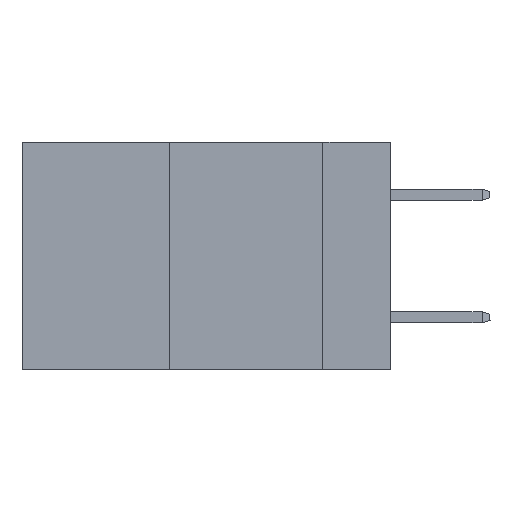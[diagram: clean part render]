
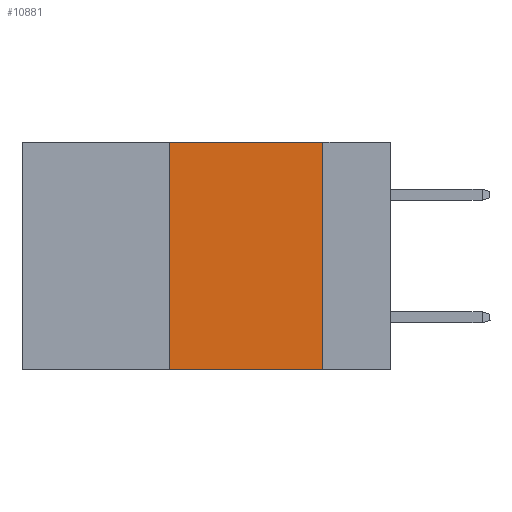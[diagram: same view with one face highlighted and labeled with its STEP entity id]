
A CAD part, left-side view. The second image highlights one B-rep face of the part: STEP entity #10881.
In plain terms, the highlighted planar face has unit normal (-1, 0, 0).
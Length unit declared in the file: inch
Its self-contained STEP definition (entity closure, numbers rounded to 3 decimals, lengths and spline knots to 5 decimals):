
#138 = DIRECTION ( 'NONE',  ( 0., -1., 0. ) ) ;
#1046 = DIRECTION ( 'NONE',  ( 0., -1., 0. ) ) ;
#1089 = VERTEX_POINT ( 'NONE', #20756 ) ;
#2280 = VERTEX_POINT ( 'NONE', #20161 ) ;
#2423 = EDGE_CURVE ( 'NONE', #1089, #2280, #5255, .T. ) ;
#2835 = PLANE ( 'NONE',  #19701 ) ;
#4960 = LINE ( 'NONE', #23471, #11288 ) ;
#5255 = LINE ( 'NONE', #24711, #20004 ) ;
#8834 = DIRECTION ( 'NONE',  ( 1., 0., 0. ) ) ;
#9177 = ORIENTED_EDGE ( 'NONE', *, *, #2423, .F. ) ;
#9410 = DIRECTION ( 'NONE',  ( 0., 0., 1. ) ) ;
#10291 = EDGE_CURVE ( 'NONE', #25453, #2280, #19579, .T. ) ;
#10881 = ADVANCED_FACE ( 'NONE', ( #21775 ), #2835, .F. ) ;
#11288 = VECTOR ( 'NONE', #9410, 39.37008 ) ;
#11901 = CARTESIAN_POINT ( 'NONE',  ( 0., 0.6, 0. ) ) ;
#12228 = ORIENTED_EDGE ( 'NONE', *, *, #10291, .T. ) ;
#12396 = LINE ( 'NONE', #11901, #24293 ) ;
#12636 = EDGE_LOOP ( 'NONE', ( #9177, #16327, #13466, #12228 ) ) ;
#13466 = ORIENTED_EDGE ( 'NONE', *, *, #22051, .F. ) ;
#16327 = ORIENTED_EDGE ( 'NONE', *, *, #21061, .F. ) ;
#16903 = CARTESIAN_POINT ( 'NONE',  ( 0., 0.6, 0. ) ) ;
#19579 = LINE ( 'NONE', #21078, #21771 ) ;
#19701 = AXIS2_PLACEMENT_3D ( 'NONE', #16903, #8834, #24838 ) ;
#20004 = VECTOR ( 'NONE', #24361, 39.37008 ) ;
#20161 = CARTESIAN_POINT ( 'NONE',  ( 0., 0.11, -0.37 ) ) ;
#20756 = CARTESIAN_POINT ( 'NONE',  ( 0., 0.11, 0. ) ) ;
#21061 = EDGE_CURVE ( 'NONE', #24851, #1089, #12396, .T. ) ;
#21078 = CARTESIAN_POINT ( 'NONE',  ( 0., 0.6, -0.37 ) ) ;
#21771 = VECTOR ( 'NONE', #1046, 39.37008 ) ;
#21775 = FACE_OUTER_BOUND ( 'NONE', #12636, .T. ) ;
#21942 = CARTESIAN_POINT ( 'NONE',  ( 0., 0.36, -0.37 ) ) ;
#22051 = EDGE_CURVE ( 'NONE', #25453, #24851, #4960, .T. ) ;
#22465 = CARTESIAN_POINT ( 'NONE',  ( 0., 0.36, 0. ) ) ;
#23471 = CARTESIAN_POINT ( 'NONE',  ( 0., 0.36, 0. ) ) ;
#24293 = VECTOR ( 'NONE', #138, 39.37008 ) ;
#24361 = DIRECTION ( 'NONE',  ( 0., 0., -1. ) ) ;
#24711 = CARTESIAN_POINT ( 'NONE',  ( 0., 0.11, 0. ) ) ;
#24838 = DIRECTION ( 'NONE',  ( 0., 0., -1. ) ) ;
#24851 = VERTEX_POINT ( 'NONE', #22465 ) ;
#25453 = VERTEX_POINT ( 'NONE', #21942 ) ;
